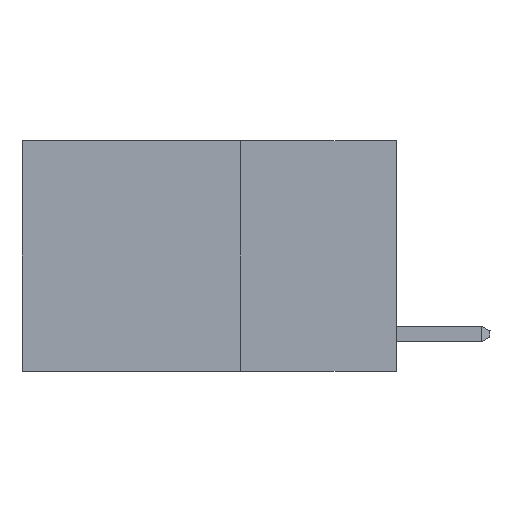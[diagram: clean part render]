
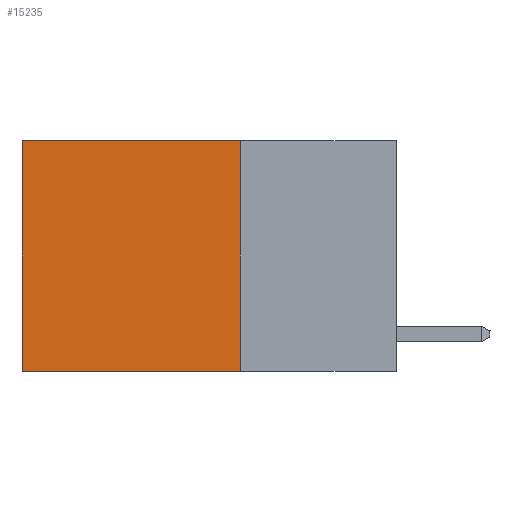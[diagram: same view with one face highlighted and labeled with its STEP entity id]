
A CAD part, left-side view. The second image highlights one B-rep face of the part: STEP entity #15235.
In plain terms, the highlighted planar face has unit normal (-1, 0, 0).
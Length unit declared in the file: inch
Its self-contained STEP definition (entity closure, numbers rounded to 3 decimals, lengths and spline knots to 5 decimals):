
#614 = CARTESIAN_POINT ( 'NONE',  ( 0.2625, 0.25, 0. ) ) ;
#728 = DIRECTION ( 'NONE',  ( 0., 0., -1. ) ) ;
#768 = DIRECTION ( 'NONE',  ( 0., 1., 0. ) ) ;
#1341 = CARTESIAN_POINT ( 'NONE',  ( 0.2625, 0.6, -0.37 ) ) ;
#1437 = LINE ( 'NONE', #8292, #13415 ) ;
#1774 = DIRECTION ( 'NONE',  ( 0., 0., -1. ) ) ;
#3408 = CARTESIAN_POINT ( 'NONE',  ( 0.2625, 0.25, 0. ) ) ;
#3411 = ORIENTED_EDGE ( 'NONE', *, *, #14138, .F. ) ;
#4842 = LINE ( 'NONE', #8988, #4906 ) ;
#4906 = VECTOR ( 'NONE', #10489, 39.37008 ) ;
#5431 = EDGE_CURVE ( 'NONE', #10499, #10045, #1437, .T. ) ;
#6449 = DIRECTION ( 'NONE',  ( 0., 0., -1. ) ) ;
#6511 = CARTESIAN_POINT ( 'NONE',  ( 0.2625, 0.25, -0.37 ) ) ;
#6765 = CARTESIAN_POINT ( 'NONE',  ( 0.2625, 0.6, 0. ) ) ;
#7390 = EDGE_CURVE ( 'NONE', #10227, #10499, #4842, .T. ) ;
#7459 = VERTEX_POINT ( 'NONE', #6511 ) ;
#8292 = CARTESIAN_POINT ( 'NONE',  ( 0.2625, 0.6, 0. ) ) ;
#8988 = CARTESIAN_POINT ( 'NONE',  ( 0.2625, 0.25, 0. ) ) ;
#9272 = FACE_OUTER_BOUND ( 'NONE', #12678, .T. ) ;
#10045 = VERTEX_POINT ( 'NONE', #1341 ) ;
#10227 = VERTEX_POINT ( 'NONE', #614 ) ;
#10368 = LINE ( 'NONE', #15708, #12617 ) ;
#10489 = DIRECTION ( 'NONE',  ( 0., 1., 0. ) ) ;
#10499 = VERTEX_POINT ( 'NONE', #6765 ) ;
#12617 = VECTOR ( 'NONE', #768, 39.37008 ) ;
#12678 = EDGE_LOOP ( 'NONE', ( #16100, #3411, #14573, #13048 ) ) ;
#13048 = ORIENTED_EDGE ( 'NONE', *, *, #7390, .T. ) ;
#13131 = DIRECTION ( 'NONE',  ( 1., 0., 0. ) ) ;
#13242 = VECTOR ( 'NONE', #728, 39.37008 ) ;
#13309 = CARTESIAN_POINT ( 'NONE',  ( 0.2625, 0.25, 0. ) ) ;
#13415 = VECTOR ( 'NONE', #1774, 39.37008 ) ;
#14138 = EDGE_CURVE ( 'NONE', #7459, #10045, #10368, .T. ) ;
#14342 = LINE ( 'NONE', #3408, #13242 ) ;
#14423 = PLANE ( 'NONE',  #15125 ) ;
#14573 = ORIENTED_EDGE ( 'NONE', *, *, #16385, .F. ) ;
#15125 = AXIS2_PLACEMENT_3D ( 'NONE', #13309, #13131, #6449 ) ;
#15235 = ADVANCED_FACE ( 'NONE', ( #9272 ), #14423, .F. ) ;
#15708 = CARTESIAN_POINT ( 'NONE',  ( 0.2625, 0.25, -0.37 ) ) ;
#16100 = ORIENTED_EDGE ( 'NONE', *, *, #5431, .T. ) ;
#16385 = EDGE_CURVE ( 'NONE', #10227, #7459, #14342, .T. ) ;
